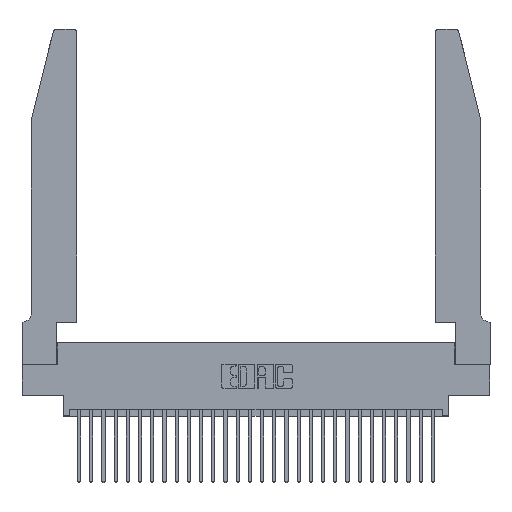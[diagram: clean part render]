
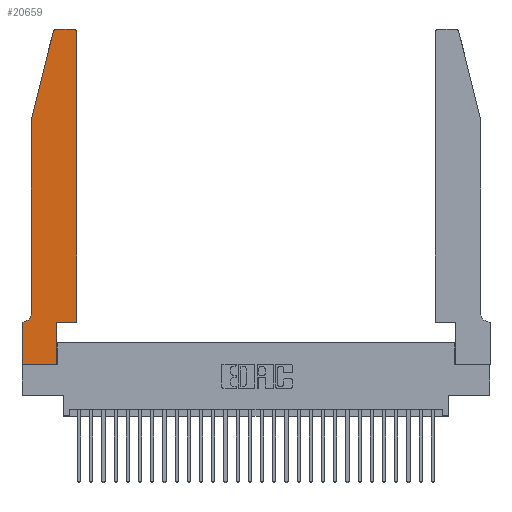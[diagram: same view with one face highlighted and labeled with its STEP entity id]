
A CAD part, top view. The second image highlights one B-rep face of the part: STEP entity #20659.
In plain terms, the highlighted planar face has unit normal (0, 0, 1).
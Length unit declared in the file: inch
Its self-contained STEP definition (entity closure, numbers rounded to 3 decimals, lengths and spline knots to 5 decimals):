
#349 = AXIS2_PLACEMENT_3D ( 'NONE', #11517, #27768, #13878 ) ;
#366 = LINE ( 'NONE', #5468, #24393 ) ;
#743 = VECTOR ( 'NONE', #26353, 39.37008 ) ;
#887 = VERTEX_POINT ( 'NONE', #3370 ) ;
#1413 = EDGE_LOOP ( 'NONE', ( #9424, #3749, #22552, #24451, #21341, #27035, #8215, #27089, #27780, #16339, #15506, #27966 ) ) ;
#1424 = CARTESIAN_POINT ( 'NONE',  ( 0., 0.35, 0.37 ) ) ;
#1493 = EDGE_CURVE ( 'NONE', #887, #16519, #366, .T. ) ;
#1918 = CARTESIAN_POINT ( 'NONE',  ( 0., 0., 0.37 ) ) ;
#2089 = LINE ( 'NONE', #1918, #26037 ) ;
#3036 = CARTESIAN_POINT ( 'NONE',  ( 0.2865, 0.35, 0.37 ) ) ;
#3295 = DIRECTION ( 'NONE',  ( -1., 0., 0. ) ) ;
#3370 = CARTESIAN_POINT ( 'NONE',  ( 0.0055, 0.35, 0.37 ) ) ;
#3507 = VECTOR ( 'NONE', #21381, 39.37008 ) ;
#3749 = ORIENTED_EDGE ( 'NONE', *, *, #28666, .T. ) ;
#3797 = DIRECTION ( 'NONE',  ( 1., 0., 0. ) ) ;
#4625 = EDGE_CURVE ( 'NONE', #10342, #10235, #13150, .T. ) ;
#4842 = DIRECTION ( 'NONE',  ( 0., 1., 0. ) ) ;
#5256 = EDGE_CURVE ( 'NONE', #16519, #14820, #27257, .T. ) ;
#5468 = CARTESIAN_POINT ( 'NONE',  ( 0.0755, 0.35, 0.37 ) ) ;
#5670 = DIRECTION ( 'NONE',  ( 0., -1., 0. ) ) ;
#6375 = CARTESIAN_POINT ( 'NONE',  ( 0.0755, 2., 0.37 ) ) ;
#6382 = LINE ( 'NONE', #3036, #24125 ) ;
#7884 = CARTESIAN_POINT ( 'NONE',  ( 0.2865, 0., 0.37 ) ) ;
#7916 = EDGE_CURVE ( 'NONE', #17243, #27895, #18100, .T. ) ;
#8082 = DIRECTION ( 'NONE',  ( 0., 0., 1. ) ) ;
#8215 = ORIENTED_EDGE ( 'NONE', *, *, #5256, .T. ) ;
#8624 = CARTESIAN_POINT ( 'NONE',  ( 0.4505, 0.35, 0.37 ) ) ;
#8889 = CIRCLE ( 'NONE', #349, 0.07 ) ;
#9074 = LINE ( 'NONE', #25881, #20693 ) ;
#9424 = ORIENTED_EDGE ( 'NONE', *, *, #14498, .T. ) ;
#9437 = DIRECTION ( 'NONE',  ( 0., 0., 1. ) ) ;
#9980 = EDGE_CURVE ( 'NONE', #22157, #12721, #15828, .T. ) ;
#10235 = VERTEX_POINT ( 'NONE', #8624 ) ;
#10342 = VERTEX_POINT ( 'NONE', #28424 ) ;
#10987 = AXIS2_PLACEMENT_3D ( 'NONE', #1424, #17704, #3797 ) ;
#11400 = EDGE_CURVE ( 'NONE', #12721, #887, #8889, .T. ) ;
#11481 = CARTESIAN_POINT ( 'NONE',  ( 0.284, 2.75, 0.37 ) ) ;
#11517 = CARTESIAN_POINT ( 'NONE',  ( 0.0055, 0.42, 0.37 ) ) ;
#12721 = VERTEX_POINT ( 'NONE', #15731 ) ;
#13014 = PLANE ( 'NONE',  #10987 ) ;
#13150 = LINE ( 'NONE', #24038, #743 ) ;
#13589 = VERTEX_POINT ( 'NONE', #7884 ) ;
#13761 = CARTESIAN_POINT ( 'NONE',  ( 0.2605, 2.75, 0.37 ) ) ;
#13795 = FACE_OUTER_BOUND ( 'NONE', #1413, .T. ) ;
#13878 = DIRECTION ( 'NONE',  ( -1., 0., 0. ) ) ;
#14498 = EDGE_CURVE ( 'NONE', #27895, #28276, #25762, .T. ) ;
#14820 = VERTEX_POINT ( 'NONE', #24101 ) ;
#15506 = ORIENTED_EDGE ( 'NONE', *, *, #24330, .T. ) ;
#15731 = CARTESIAN_POINT ( 'NONE',  ( 0.0755, 0.42, 0.37 ) ) ;
#15828 = LINE ( 'NONE', #19093, #3507 ) ;
#16078 = DIRECTION ( 'NONE',  ( -1., 0., 0. ) ) ;
#16339 = ORIENTED_EDGE ( 'NONE', *, *, #4625, .T. ) ;
#16519 = VERTEX_POINT ( 'NONE', #26317 ) ;
#16934 = DIRECTION ( 'NONE',  ( 0., 1., 0. ) ) ;
#17089 = VECTOR ( 'NONE', #4842, 39.37008 ) ;
#17243 = VERTEX_POINT ( 'NONE', #22129 ) ;
#17361 = AXIS2_PLACEMENT_3D ( 'NONE', #21943, #8082, #24275 ) ;
#17704 = DIRECTION ( 'NONE',  ( 0., 0., 1. ) ) ;
#18100 = CIRCLE ( 'NONE', #19262, 0.03 ) ;
#19093 = CARTESIAN_POINT ( 'NONE',  ( 0.0755, 2., 0.37 ) ) ;
#19189 = CARTESIAN_POINT ( 'NONE',  ( 0.4205, 2.75, 0.37 ) ) ;
#19262 = AXIS2_PLACEMENT_3D ( 'NONE', #23309, #9437, #25631 ) ;
#20396 = VECTOR ( 'NONE', #5670, 39.37008 ) ;
#20422 = VERTEX_POINT ( 'NONE', #21550 ) ;
#20659 = ADVANCED_FACE ( 'NONE', ( #13795 ), #13014, .T. ) ;
#20693 = VECTOR ( 'NONE', #28208, 39.37008 ) ;
#21341 = ORIENTED_EDGE ( 'NONE', *, *, #11400, .T. ) ;
#21381 = DIRECTION ( 'NONE',  ( 0., -1., 0. ) ) ;
#21550 = CARTESIAN_POINT ( 'NONE',  ( 0.25487, 2.72718, 0.37 ) ) ;
#21731 = CIRCLE ( 'NONE', #17361, 0.03 ) ;
#21943 = CARTESIAN_POINT ( 'NONE',  ( 0.284, 2.72, 0.37 ) ) ;
#22129 = CARTESIAN_POINT ( 'NONE',  ( 0.4505, 2.72, 0.37 ) ) ;
#22157 = VERTEX_POINT ( 'NONE', #6375 ) ;
#22552 = ORIENTED_EDGE ( 'NONE', *, *, #25122, .T. ) ;
#22840 = DIRECTION ( 'NONE',  ( 1., 0., 0. ) ) ;
#23237 = LINE ( 'NONE', #27811, #17089 ) ;
#23309 = CARTESIAN_POINT ( 'NONE',  ( 0.4205, 2.72, 0.37 ) ) ;
#24038 = CARTESIAN_POINT ( 'NONE',  ( 0.4505, 0.35, 0.37 ) ) ;
#24101 = CARTESIAN_POINT ( 'NONE',  ( 0., 0., 0.37 ) ) ;
#24125 = VECTOR ( 'NONE', #16934, 39.37008 ) ;
#24275 = DIRECTION ( 'NONE',  ( 1., 0., 0. ) ) ;
#24330 = EDGE_CURVE ( 'NONE', #10235, #17243, #23237, .T. ) ;
#24332 = VECTOR ( 'NONE', #16078, 39.37008 ) ;
#24393 = VECTOR ( 'NONE', #3295, 39.37008 ) ;
#24451 = ORIENTED_EDGE ( 'NONE', *, *, #9980, .T. ) ;
#25122 = EDGE_CURVE ( 'NONE', #20422, #22157, #9074, .T. ) ;
#25631 = DIRECTION ( 'NONE',  ( 1., 0., 0. ) ) ;
#25762 = LINE ( 'NONE', #13761, #24332 ) ;
#25881 = CARTESIAN_POINT ( 'NONE',  ( 0.0755, 2., 0.37 ) ) ;
#26037 = VECTOR ( 'NONE', #22840, 39.37008 ) ;
#26317 = CARTESIAN_POINT ( 'NONE',  ( 0., 0.35, 0.37 ) ) ;
#26353 = DIRECTION ( 'NONE',  ( 1., 0., 0. ) ) ;
#27035 = ORIENTED_EDGE ( 'NONE', *, *, #1493, .T. ) ;
#27089 = ORIENTED_EDGE ( 'NONE', *, *, #28926, .T. ) ;
#27257 = LINE ( 'NONE', #28617, #20396 ) ;
#27768 = DIRECTION ( 'NONE',  ( 0., 0., -1. ) ) ;
#27780 = ORIENTED_EDGE ( 'NONE', *, *, #27815, .T. ) ;
#27811 = CARTESIAN_POINT ( 'NONE',  ( 0.4505, 0.35, 0.37 ) ) ;
#27815 = EDGE_CURVE ( 'NONE', #13589, #10342, #6382, .T. ) ;
#27895 = VERTEX_POINT ( 'NONE', #19189 ) ;
#27966 = ORIENTED_EDGE ( 'NONE', *, *, #7916, .T. ) ;
#28208 = DIRECTION ( 'NONE',  ( -0.239, -0.971, 0. ) ) ;
#28276 = VERTEX_POINT ( 'NONE', #11481 ) ;
#28424 = CARTESIAN_POINT ( 'NONE',  ( 0.2865, 0.35, 0.37 ) ) ;
#28617 = CARTESIAN_POINT ( 'NONE',  ( 0., 0., 0.37 ) ) ;
#28666 = EDGE_CURVE ( 'NONE', #28276, #20422, #21731, .T. ) ;
#28926 = EDGE_CURVE ( 'NONE', #14820, #13589, #2089, .T. ) ;
